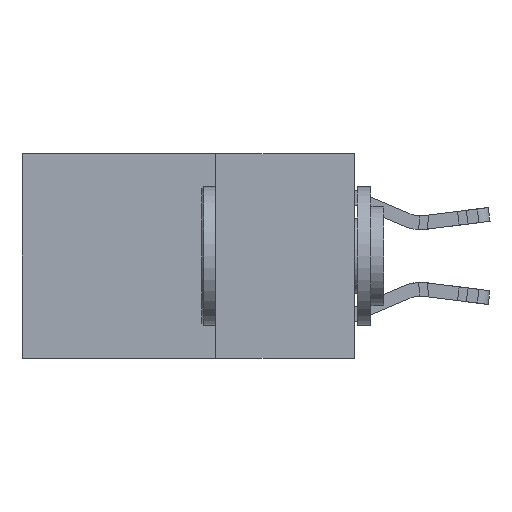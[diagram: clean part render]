
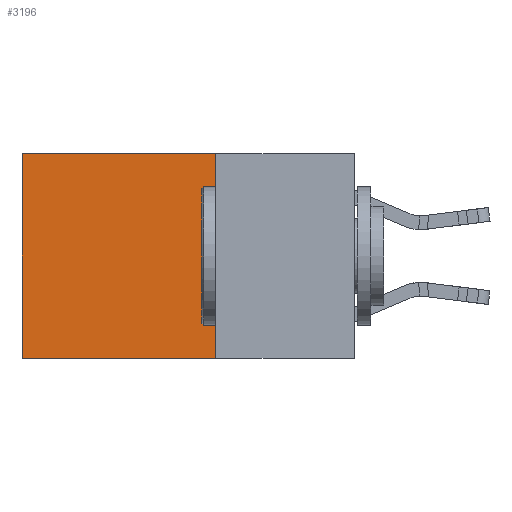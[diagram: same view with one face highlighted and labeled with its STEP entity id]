
A CAD part, left-side view. The second image highlights one B-rep face of the part: STEP entity #3196.
In plain terms, the highlighted planar face has unit normal (-1, 0, 0).
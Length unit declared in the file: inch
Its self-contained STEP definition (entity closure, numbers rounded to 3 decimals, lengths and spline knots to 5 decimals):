
#1335 = DIRECTION ( 'NONE',  ( 0., 1., 0. ) ) ;
#2906 = ORIENTED_EDGE ( 'NONE', *, *, #28482, .F. ) ;
#3196 = ADVANCED_FACE ( 'NONE', ( #20908 ), #15443, .F. ) ;
#3570 = CARTESIAN_POINT ( 'NONE',  ( 0.2625, 0.25, 0. ) ) ;
#3620 = VECTOR ( 'NONE', #24804, 39.37008 ) ;
#4407 = CARTESIAN_POINT ( 'NONE',  ( 0.2625, 0.6, 0. ) ) ;
#8320 = CARTESIAN_POINT ( 'NONE',  ( 0.2625, 0.25, -0.37 ) ) ;
#9828 = ORIENTED_EDGE ( 'NONE', *, *, #27984, .T. ) ;
#10262 = VECTOR ( 'NONE', #24069, 39.37008 ) ;
#10441 = EDGE_LOOP ( 'NONE', ( #10739, #29694, #2906, #9828 ) ) ;
#10739 = ORIENTED_EDGE ( 'NONE', *, *, #18753, .T. ) ;
#10746 = DIRECTION ( 'NONE',  ( 0., 0., -1. ) ) ;
#13431 = VERTEX_POINT ( 'NONE', #30236 ) ;
#14651 = AXIS2_PLACEMENT_3D ( 'NONE', #24788, #24885, #10746 ) ;
#15443 = PLANE ( 'NONE',  #14651 ) ;
#17092 = LINE ( 'NONE', #4407, #29583 ) ;
#17414 = EDGE_CURVE ( 'NONE', #19349, #30154, #28230, .T. ) ;
#18753 = EDGE_CURVE ( 'NONE', #20473, #30154, #17092, .T. ) ;
#19342 = CARTESIAN_POINT ( 'NONE',  ( 0.2625, 0.25, 0. ) ) ;
#19349 = VERTEX_POINT ( 'NONE', #20346 ) ;
#20346 = CARTESIAN_POINT ( 'NONE',  ( 0.2625, 0.25, -0.37 ) ) ;
#20473 = VERTEX_POINT ( 'NONE', #28947 ) ;
#20908 = FACE_OUTER_BOUND ( 'NONE', #10441, .T. ) ;
#21953 = VECTOR ( 'NONE', #1335, 39.37008 ) ;
#23235 = DIRECTION ( 'NONE',  ( 0., 0., -1. ) ) ;
#24069 = DIRECTION ( 'NONE',  ( 0., 0., -1. ) ) ;
#24788 = CARTESIAN_POINT ( 'NONE',  ( 0.2625, 0.25, 0. ) ) ;
#24804 = DIRECTION ( 'NONE',  ( 0., 1., 0. ) ) ;
#24885 = DIRECTION ( 'NONE',  ( 1., 0., 0. ) ) ;
#27984 = EDGE_CURVE ( 'NONE', #13431, #20473, #28688, .T. ) ;
#27995 = CARTESIAN_POINT ( 'NONE',  ( 0.2625, 0.6, -0.37 ) ) ;
#28230 = LINE ( 'NONE', #8320, #21953 ) ;
#28482 = EDGE_CURVE ( 'NONE', #13431, #19349, #29092, .T. ) ;
#28688 = LINE ( 'NONE', #3570, #3620 ) ;
#28947 = CARTESIAN_POINT ( 'NONE',  ( 0.2625, 0.6, 0. ) ) ;
#29092 = LINE ( 'NONE', #19342, #10262 ) ;
#29583 = VECTOR ( 'NONE', #23235, 39.37008 ) ;
#29694 = ORIENTED_EDGE ( 'NONE', *, *, #17414, .F. ) ;
#30154 = VERTEX_POINT ( 'NONE', #27995 ) ;
#30236 = CARTESIAN_POINT ( 'NONE',  ( 0.2625, 0.25, 0. ) ) ;
